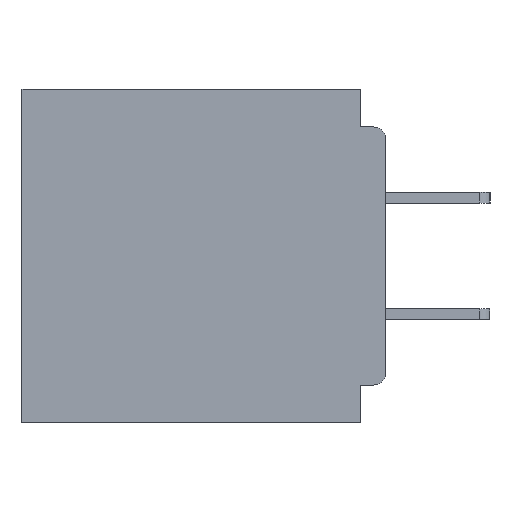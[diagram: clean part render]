
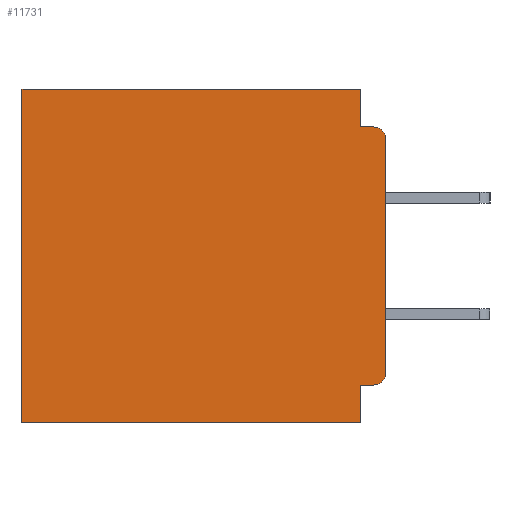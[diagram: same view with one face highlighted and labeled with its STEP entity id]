
A CAD part, left-side view. The second image highlights one B-rep face of the part: STEP entity #11731.
In plain terms, the highlighted planar face has unit normal (-1, 0, 0).
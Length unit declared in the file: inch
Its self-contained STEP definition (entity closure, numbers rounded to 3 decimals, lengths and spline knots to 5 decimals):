
#210 = CARTESIAN_POINT ( 'NONE',  ( 0.3, 0.031, -0.4 ) ) ;
#456 = VERTEX_POINT ( 'NONE', #22788 ) ;
#603 = VERTEX_POINT ( 'NONE', #20421 ) ;
#627 = EDGE_CURVE ( 'NONE', #4573, #37287, #6621, .T. ) ;
#1187 = ORIENTED_EDGE ( 'NONE', *, *, #7499, .T. ) ;
#3030 = ORIENTED_EDGE ( 'NONE', *, *, #26148, .F. ) ;
#3101 = CARTESIAN_POINT ( 'NONE',  ( 0.3, 0., -0.4 ) ) ;
#4217 = EDGE_CURVE ( 'NONE', #22825, #18389, #22189, .T. ) ;
#4573 = VERTEX_POINT ( 'NONE', #9548 ) ;
#4972 = DIRECTION ( 'NONE',  ( 0., 0., -1. ) ) ;
#5665 = VECTOR ( 'NONE', #4972, 39.37008 ) ;
#5746 = VECTOR ( 'NONE', #18277, 39.37008 ) ;
#6621 = LINE ( 'NONE', #7155, #5665 ) ;
#7155 = CARTESIAN_POINT ( 'NONE',  ( 0.3, 0.031, -0.4 ) ) ;
#7499 = EDGE_CURVE ( 'NONE', #14421, #11529, #24627, .T. ) ;
#7573 = LINE ( 'NONE', #21897, #13828 ) ;
#8625 = EDGE_LOOP ( 'NONE', ( #16850, #35872, #3030, #24807, #21016, #12939, #17511, #10045, #16823, #1187 ) ) ;
#8703 = VECTOR ( 'NONE', #18367, 39.37008 ) ;
#9548 = CARTESIAN_POINT ( 'NONE',  ( 0.3, 0.031, -0.355 ) ) ;
#10045 = ORIENTED_EDGE ( 'NONE', *, *, #627, .F. ) ;
#10607 = VERTEX_POINT ( 'NONE', #20444 ) ;
#11312 = LINE ( 'NONE', #31114, #19473 ) ;
#11529 = VERTEX_POINT ( 'NONE', #18503 ) ;
#11731 = ADVANCED_FACE ( 'NONE', ( #34387 ), #16495, .F. ) ;
#11881 = VECTOR ( 'NONE', #15992, 39.37008 ) ;
#12405 = CARTESIAN_POINT ( 'NONE',  ( 0.3, 0., -0.045 ) ) ;
#12756 = DIRECTION ( 'NONE',  ( 0., 1., 0. ) ) ;
#12903 = CARTESIAN_POINT ( 'NONE',  ( 0.3, 0., -0.4 ) ) ;
#12939 = ORIENTED_EDGE ( 'NONE', *, *, #17106, .T. ) ;
#13828 = VECTOR ( 'NONE', #34095, 39.37008 ) ;
#14421 = VERTEX_POINT ( 'NONE', #35387 ) ;
#15497 = DIRECTION ( 'NONE',  ( 0., -1., 0. ) ) ;
#15613 = AXIS2_PLACEMENT_3D ( 'NONE', #17073, #38534, #20143 ) ;
#15992 = DIRECTION ( 'NONE',  ( 0., 1., 0. ) ) ;
#16495 = PLANE ( 'NONE',  #18505 ) ;
#16823 = ORIENTED_EDGE ( 'NONE', *, *, #36672, .F. ) ;
#16850 = ORIENTED_EDGE ( 'NONE', *, *, #23530, .F. ) ;
#17073 = CARTESIAN_POINT ( 'NONE',  ( 0.3, 0.015, -0.34 ) ) ;
#17106 = EDGE_CURVE ( 'NONE', #10607, #456, #25020, .T. ) ;
#17511 = ORIENTED_EDGE ( 'NONE', *, *, #28770, .F. ) ;
#18277 = DIRECTION ( 'NONE',  ( 0., 1., 0. ) ) ;
#18367 = DIRECTION ( 'NONE',  ( 0., 0., -1. ) ) ;
#18389 = VERTEX_POINT ( 'NONE', #39497 ) ;
#18435 = EDGE_CURVE ( 'NONE', #38410, #10607, #30243, .T. ) ;
#18503 = CARTESIAN_POINT ( 'NONE',  ( 0.3, 0., -0.34 ) ) ;
#18505 = AXIS2_PLACEMENT_3D ( 'NONE', #31773, #37942, #19570 ) ;
#19473 = VECTOR ( 'NONE', #12756, 39.37008 ) ;
#19570 = DIRECTION ( 'NONE',  ( 0., 0., -1. ) ) ;
#20143 = DIRECTION ( 'NONE',  ( 0., 0., -1. ) ) ;
#20421 = CARTESIAN_POINT ( 'NONE',  ( 0.3, 0.031, -0.045 ) ) ;
#20444 = CARTESIAN_POINT ( 'NONE',  ( 0.3, 0.437, 0. ) ) ;
#21016 = ORIENTED_EDGE ( 'NONE', *, *, #18435, .T. ) ;
#21363 = AXIS2_PLACEMENT_3D ( 'NONE', #27519, #27559, #27606 ) ;
#21470 = DIRECTION ( 'NONE',  ( 0., 0., -1. ) ) ;
#21897 = CARTESIAN_POINT ( 'NONE',  ( 0.3, 0.031, 0. ) ) ;
#22189 = CIRCLE ( 'NONE', #21363, 0.015 ) ;
#22788 = CARTESIAN_POINT ( 'NONE',  ( 0.3, 0.437, -0.4 ) ) ;
#22825 = VERTEX_POINT ( 'NONE', #24217 ) ;
#23530 = EDGE_CURVE ( 'NONE', #22825, #11529, #26918, .T. ) ;
#24217 = CARTESIAN_POINT ( 'NONE',  ( 0.3, 0., -0.06 ) ) ;
#24460 = CARTESIAN_POINT ( 'NONE',  ( 0.3, 0., 0. ) ) ;
#24627 = CIRCLE ( 'NONE', #15613, 0.015 ) ;
#24807 = ORIENTED_EDGE ( 'NONE', *, *, #28091, .F. ) ;
#25020 = LINE ( 'NONE', #30598, #8703 ) ;
#26148 = EDGE_CURVE ( 'NONE', #603, #18389, #28866, .T. ) ;
#26918 = LINE ( 'NONE', #3101, #35053 ) ;
#27519 = CARTESIAN_POINT ( 'NONE',  ( 0.3, 0.015, -0.06 ) ) ;
#27559 = DIRECTION ( 'NONE',  ( -1., 0., 0. ) ) ;
#27606 = DIRECTION ( 'NONE',  ( 0., 0., -1. ) ) ;
#27890 = VECTOR ( 'NONE', #15497, 39.37008 ) ;
#28091 = EDGE_CURVE ( 'NONE', #38410, #603, #7573, .T. ) ;
#28770 = EDGE_CURVE ( 'NONE', #37287, #456, #36337, .T. ) ;
#28866 = LINE ( 'NONE', #12405, #27890 ) ;
#30243 = LINE ( 'NONE', #24460, #5746 ) ;
#30598 = CARTESIAN_POINT ( 'NONE',  ( 0.3, 0.437, -0.4 ) ) ;
#31114 = CARTESIAN_POINT ( 'NONE',  ( 0.3, 0., -0.355 ) ) ;
#31773 = CARTESIAN_POINT ( 'NONE',  ( 0.3, 0., -0.4 ) ) ;
#33511 = CARTESIAN_POINT ( 'NONE',  ( 0.3, 0.031, 0. ) ) ;
#34095 = DIRECTION ( 'NONE',  ( 0., 0., -1. ) ) ;
#34387 = FACE_OUTER_BOUND ( 'NONE', #8625, .T. ) ;
#35053 = VECTOR ( 'NONE', #21470, 39.37008 ) ;
#35387 = CARTESIAN_POINT ( 'NONE',  ( 0.3, 0.015, -0.355 ) ) ;
#35872 = ORIENTED_EDGE ( 'NONE', *, *, #4217, .T. ) ;
#36337 = LINE ( 'NONE', #12903, #11881 ) ;
#36672 = EDGE_CURVE ( 'NONE', #14421, #4573, #11312, .T. ) ;
#37287 = VERTEX_POINT ( 'NONE', #210 ) ;
#37942 = DIRECTION ( 'NONE',  ( 1., 0., 0. ) ) ;
#38410 = VERTEX_POINT ( 'NONE', #33511 ) ;
#38534 = DIRECTION ( 'NONE',  ( -1., 0., 0. ) ) ;
#39497 = CARTESIAN_POINT ( 'NONE',  ( 0.3, 0.015, -0.045 ) ) ;
